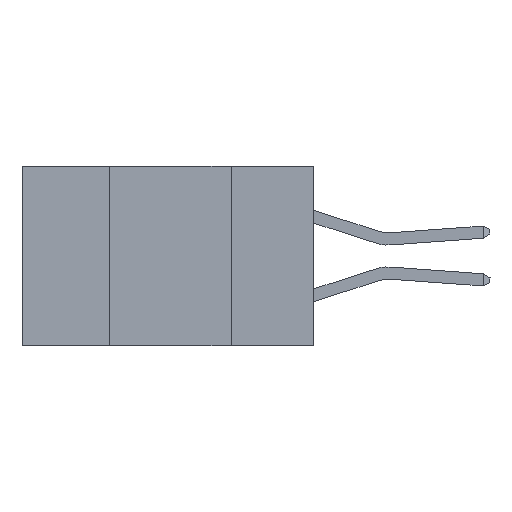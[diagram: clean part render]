
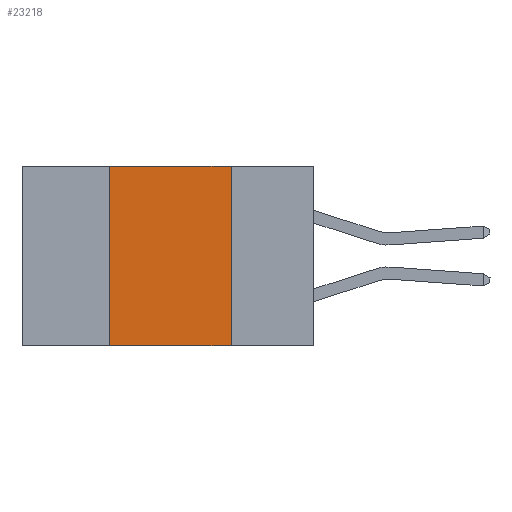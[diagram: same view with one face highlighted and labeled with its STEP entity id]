
A CAD part, left-side view. The second image highlights one B-rep face of the part: STEP entity #23218.
In plain terms, the highlighted planar face has unit normal (-1, 0, 0).
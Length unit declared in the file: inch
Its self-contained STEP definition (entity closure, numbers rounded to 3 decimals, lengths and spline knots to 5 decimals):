
#68 = CARTESIAN_POINT ( 'NONE',  ( 0., 0.42, 0. ) ) ;
#508 = VERTEX_POINT ( 'NONE', #8345 ) ;
#1657 = VECTOR ( 'NONE', #15315, 39.37008 ) ;
#3141 = DIRECTION ( 'NONE',  ( 0., 0., -1. ) ) ;
#3175 = VECTOR ( 'NONE', #10388, 39.37008 ) ;
#3316 = CARTESIAN_POINT ( 'NONE',  ( 0., 0.6, 0. ) ) ;
#4532 = DIRECTION ( 'NONE',  ( 0., -1., 0. ) ) ;
#5199 = FACE_OUTER_BOUND ( 'NONE', #18147, .T. ) ;
#5595 = ORIENTED_EDGE ( 'NONE', *, *, #6271, .F. ) ;
#6271 = EDGE_CURVE ( 'NONE', #14423, #20138, #7474, .T. ) ;
#6579 = EDGE_CURVE ( 'NONE', #508, #22900, #15202, .T. ) ;
#7474 = LINE ( 'NONE', #13329, #1657 ) ;
#8345 = CARTESIAN_POINT ( 'NONE',  ( 0., 0.17, 0. ) ) ;
#8607 = CARTESIAN_POINT ( 'NONE',  ( 0., 0.6, 0. ) ) ;
#9756 = CARTESIAN_POINT ( 'NONE',  ( 0., 0.6, -0.37 ) ) ;
#10388 = DIRECTION ( 'NONE',  ( 0., -1., 0. ) ) ;
#10540 = PLANE ( 'NONE',  #19012 ) ;
#11315 = LINE ( 'NONE', #9756, #15602 ) ;
#12045 = ORIENTED_EDGE ( 'NONE', *, *, #15177, .F. ) ;
#12222 = CARTESIAN_POINT ( 'NONE',  ( 0., 0.42, -0.37 ) ) ;
#12370 = DIRECTION ( 'NONE',  ( 1., 0., 0. ) ) ;
#13329 = CARTESIAN_POINT ( 'NONE',  ( 0., 0.42, 0. ) ) ;
#13500 = ORIENTED_EDGE ( 'NONE', *, *, #6579, .F. ) ;
#13618 = ORIENTED_EDGE ( 'NONE', *, *, #19079, .T. ) ;
#14159 = LINE ( 'NONE', #8607, #3175 ) ;
#14423 = VERTEX_POINT ( 'NONE', #12222 ) ;
#15177 = EDGE_CURVE ( 'NONE', #20138, #508, #14159, .T. ) ;
#15202 = LINE ( 'NONE', #22381, #20762 ) ;
#15315 = DIRECTION ( 'NONE',  ( 0., 0., 1. ) ) ;
#15602 = VECTOR ( 'NONE', #4532, 39.37008 ) ;
#18147 = EDGE_LOOP ( 'NONE', ( #13500, #12045, #5595, #13618 ) ) ;
#18218 = CARTESIAN_POINT ( 'NONE',  ( 0., 0.17, -0.37 ) ) ;
#19012 = AXIS2_PLACEMENT_3D ( 'NONE', #3316, #12370, #3141 ) ;
#19035 = DIRECTION ( 'NONE',  ( 0., 0., -1. ) ) ;
#19079 = EDGE_CURVE ( 'NONE', #14423, #22900, #11315, .T. ) ;
#20138 = VERTEX_POINT ( 'NONE', #68 ) ;
#20762 = VECTOR ( 'NONE', #19035, 39.37008 ) ;
#22381 = CARTESIAN_POINT ( 'NONE',  ( 0., 0.17, 0. ) ) ;
#22900 = VERTEX_POINT ( 'NONE', #18218 ) ;
#23218 = ADVANCED_FACE ( 'NONE', ( #5199 ), #10540, .F. ) ;
